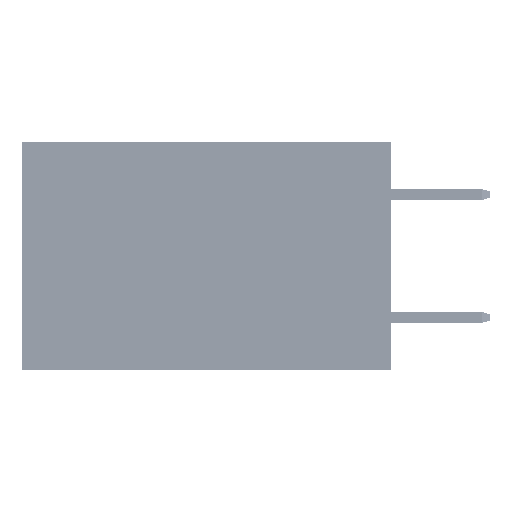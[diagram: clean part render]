
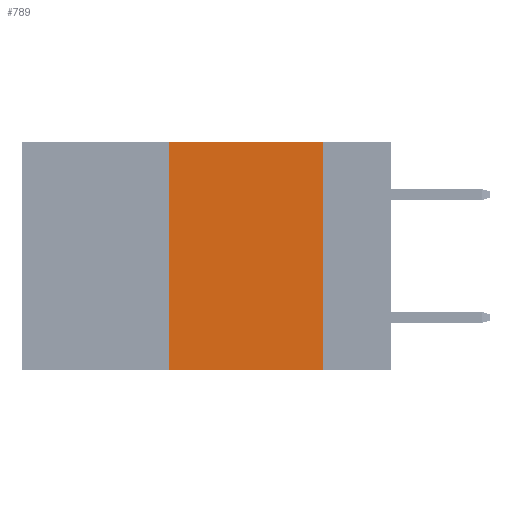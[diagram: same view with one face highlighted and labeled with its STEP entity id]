
A CAD part, left-side view. The second image highlights one B-rep face of the part: STEP entity #789.
In plain terms, the highlighted planar face has unit normal (-1, 0, 0).
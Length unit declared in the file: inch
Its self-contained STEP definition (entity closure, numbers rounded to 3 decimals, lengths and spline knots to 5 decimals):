
#496 = EDGE_CURVE ( 'NONE', #16830, #7094, #31375, .T. ) ;
#610 = CARTESIAN_POINT ( 'NONE',  ( 0., 0.11, -0.37 ) ) ;
#789 = ADVANCED_FACE ( 'NONE', ( #30119 ), #40293, .F. ) ;
#3147 = CARTESIAN_POINT ( 'NONE',  ( 0., 0.36, 0. ) ) ;
#5230 = ORIENTED_EDGE ( 'NONE', *, *, #35824, .F. ) ;
#6693 = EDGE_CURVE ( 'NONE', #16830, #38510, #26614, .T. ) ;
#7094 = VERTEX_POINT ( 'NONE', #33934 ) ;
#8881 = DIRECTION ( 'NONE',  ( 1., 0., 0. ) ) ;
#8984 = LINE ( 'NONE', #48807, #25964 ) ;
#12854 = EDGE_LOOP ( 'NONE', ( #38185, #5230, #42300, #27501 ) ) ;
#13348 = VERTEX_POINT ( 'NONE', #31141 ) ;
#16090 = DIRECTION ( 'NONE',  ( 0., -1., 0. ) ) ;
#16830 = VERTEX_POINT ( 'NONE', #27142 ) ;
#19201 = DIRECTION ( 'NONE',  ( 0., 0., -1. ) ) ;
#25964 = VECTOR ( 'NONE', #40663, 39.37008 ) ;
#26614 = LINE ( 'NONE', #43301, #37428 ) ;
#26730 = EDGE_CURVE ( 'NONE', #13348, #38510, #27653, .T. ) ;
#27142 = CARTESIAN_POINT ( 'NONE',  ( 0., 0.36, -0.37 ) ) ;
#27501 = ORIENTED_EDGE ( 'NONE', *, *, #6693, .T. ) ;
#27653 = LINE ( 'NONE', #45905, #37891 ) ;
#29927 = AXIS2_PLACEMENT_3D ( 'NONE', #44208, #8881, #36052 ) ;
#30119 = FACE_OUTER_BOUND ( 'NONE', #12854, .T. ) ;
#31141 = CARTESIAN_POINT ( 'NONE',  ( 0., 0.11, 0. ) ) ;
#31375 = LINE ( 'NONE', #3147, #36163 ) ;
#33934 = CARTESIAN_POINT ( 'NONE',  ( 0., 0.36, 0. ) ) ;
#35824 = EDGE_CURVE ( 'NONE', #7094, #13348, #8984, .T. ) ;
#36052 = DIRECTION ( 'NONE',  ( 0., 0., -1. ) ) ;
#36163 = VECTOR ( 'NONE', #42212, 39.37008 ) ;
#37428 = VECTOR ( 'NONE', #16090, 39.37008 ) ;
#37891 = VECTOR ( 'NONE', #19201, 39.37008 ) ;
#38185 = ORIENTED_EDGE ( 'NONE', *, *, #26730, .F. ) ;
#38510 = VERTEX_POINT ( 'NONE', #610 ) ;
#40293 = PLANE ( 'NONE',  #29927 ) ;
#40663 = DIRECTION ( 'NONE',  ( 0., -1., 0. ) ) ;
#42212 = DIRECTION ( 'NONE',  ( 0., 0., 1. ) ) ;
#42300 = ORIENTED_EDGE ( 'NONE', *, *, #496, .F. ) ;
#43301 = CARTESIAN_POINT ( 'NONE',  ( 0., 0.6, -0.37 ) ) ;
#44208 = CARTESIAN_POINT ( 'NONE',  ( 0., 0.6, 0. ) ) ;
#45905 = CARTESIAN_POINT ( 'NONE',  ( 0., 0.11, 0. ) ) ;
#48807 = CARTESIAN_POINT ( 'NONE',  ( 0., 0.6, 0. ) ) ;
